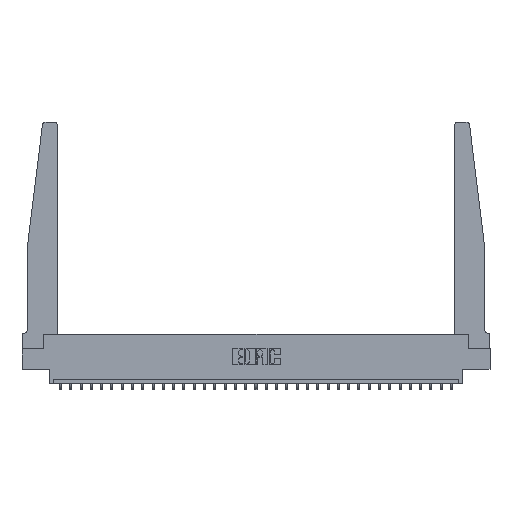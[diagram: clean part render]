
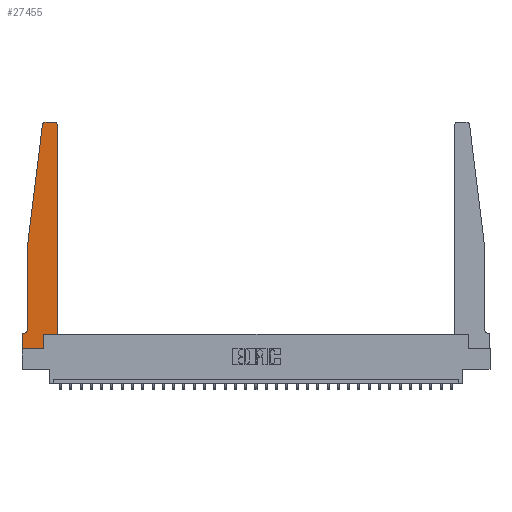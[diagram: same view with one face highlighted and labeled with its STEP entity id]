
A CAD part, top view. The second image highlights one B-rep face of the part: STEP entity #27455.
In plain terms, the highlighted planar face has unit normal (0, 0, 1).
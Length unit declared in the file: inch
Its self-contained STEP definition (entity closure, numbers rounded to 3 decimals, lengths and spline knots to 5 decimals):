
#43 = CARTESIAN_POINT ( 'NONE',  ( 0.065, 0.2375, 0.37 ) ) ;
#431 = CARTESIAN_POINT ( 'NONE',  ( 0.2605, 0., 0.37 ) ) ;
#449 = CARTESIAN_POINT ( 'NONE',  ( 0.395, 2.72, 0.37 ) ) ;
#1657 = AXIS2_PLACEMENT_3D ( 'NONE', #6123, #22128, #8421 ) ;
#2112 = CARTESIAN_POINT ( 'NONE',  ( 0.395, 2.75, 0.37 ) ) ;
#2204 = PLANE ( 'NONE',  #16980 ) ;
#2586 = CARTESIAN_POINT ( 'NONE',  ( 0.015, 0.2375, 0.37 ) ) ;
#2654 = DIRECTION ( 'NONE',  ( 0., -1., 0. ) ) ;
#2761 = DIRECTION ( 'NONE',  ( 1., 0., 0. ) ) ;
#3505 = VERTEX_POINT ( 'NONE', #2112 ) ;
#3593 = DIRECTION ( 'NONE',  ( 1., 0., 0. ) ) ;
#3623 = ORIENTED_EDGE ( 'NONE', *, *, #20259, .T. ) ;
#3693 = CARTESIAN_POINT ( 'NONE',  ( 0.425, 0.18, 0.37 ) ) ;
#3745 = CARTESIAN_POINT ( 'NONE',  ( 0.425, 2.72, 0.37 ) ) ;
#3950 = LINE ( 'NONE', #18635, #22200 ) ;
#3985 = EDGE_LOOP ( 'NONE', ( #28343, #24092, #12343, #15617, #10649, #20287, #22351, #16852, #3623, #20044, #4111, #4982 ) ) ;
#4071 = VERTEX_POINT ( 'NONE', #15637 ) ;
#4111 = ORIENTED_EDGE ( 'NONE', *, *, #15782, .T. ) ;
#4496 = EDGE_CURVE ( 'NONE', #15109, #15388, #22783, .T. ) ;
#4830 = DIRECTION ( 'NONE',  ( -1., 0., 0. ) ) ;
#4880 = VECTOR ( 'NONE', #12993, 39.37008 ) ;
#4982 = ORIENTED_EDGE ( 'NONE', *, *, #11538, .T. ) ;
#5104 = EDGE_CURVE ( 'NONE', #25351, #8278, #6281, .T. ) ;
#5552 = VERTEX_POINT ( 'NONE', #13343 ) ;
#5752 = CARTESIAN_POINT ( 'NONE',  ( 0., 0., 0.37 ) ) ;
#6123 = CARTESIAN_POINT ( 'NONE',  ( 0.27653, 2.72, 0.37 ) ) ;
#6281 = CIRCLE ( 'NONE', #25592, 0.05 ) ;
#6567 = LINE ( 'NONE', #28541, #11937 ) ;
#6596 = LINE ( 'NONE', #3693, #16604 ) ;
#6695 = VERTEX_POINT ( 'NONE', #15187 ) ;
#6770 = DIRECTION ( 'NONE',  ( 0., 0., 1. ) ) ;
#6935 = DIRECTION ( 'NONE',  ( -0.122, -0.992, 0. ) ) ;
#6980 = CARTESIAN_POINT ( 'NONE',  ( 0.2605, 0.18, 0.37 ) ) ;
#7722 = CARTESIAN_POINT ( 'NONE',  ( 0., 0.1875, 0.37 ) ) ;
#7790 = EDGE_CURVE ( 'NONE', #15388, #5552, #26459, .T. ) ;
#8278 = VERTEX_POINT ( 'NONE', #27007 ) ;
#8357 = DIRECTION ( 'NONE',  ( -1., 0., 0. ) ) ;
#8410 = CARTESIAN_POINT ( 'NONE',  ( 0.27653, 2.75, 0.37 ) ) ;
#8421 = DIRECTION ( 'NONE',  ( 1., 0., 0. ) ) ;
#8904 = EDGE_CURVE ( 'NONE', #11662, #17621, #9171, .T. ) ;
#9171 = LINE ( 'NONE', #29138, #21384 ) ;
#10018 = AXIS2_PLACEMENT_3D ( 'NONE', #449, #16435, #2761 ) ;
#10250 = DIRECTION ( 'NONE',  ( -1., 0., 0. ) ) ;
#10649 = ORIENTED_EDGE ( 'NONE', *, *, #5104, .T. ) ;
#11099 = EDGE_CURVE ( 'NONE', #8278, #11662, #6567, .T. ) ;
#11213 = EDGE_CURVE ( 'NONE', #3505, #15109, #21251, .T. ) ;
#11538 = EDGE_CURVE ( 'NONE', #25711, #3505, #13349, .T. ) ;
#11596 = DIRECTION ( 'NONE',  ( 0., 1., 0. ) ) ;
#11662 = VERTEX_POINT ( 'NONE', #7722 ) ;
#11937 = VECTOR ( 'NONE', #10250, 39.37008 ) ;
#12343 = ORIENTED_EDGE ( 'NONE', *, *, #7790, .T. ) ;
#12993 = DIRECTION ( 'NONE',  ( 0., 1., 0. ) ) ;
#13343 = CARTESIAN_POINT ( 'NONE',  ( 0.065, 1.25, 0.37 ) ) ;
#13349 = CIRCLE ( 'NONE', #10018, 0.03 ) ;
#13579 = VECTOR ( 'NONE', #6935, 39.37008 ) ;
#15109 = VERTEX_POINT ( 'NONE', #8410 ) ;
#15187 = CARTESIAN_POINT ( 'NONE',  ( 0.2605, 0.18, 0.37 ) ) ;
#15189 = CARTESIAN_POINT ( 'NONE',  ( 0.425, 0.18, 0.37 ) ) ;
#15388 = VERTEX_POINT ( 'NONE', #16288 ) ;
#15478 = DIRECTION ( 'NONE',  ( 0., -1., 0. ) ) ;
#15617 = ORIENTED_EDGE ( 'NONE', *, *, #28220, .T. ) ;
#15637 = CARTESIAN_POINT ( 'NONE',  ( 0.425, 0.18, 0.37 ) ) ;
#15782 = EDGE_CURVE ( 'NONE', #4071, #25711, #23158, .T. ) ;
#16288 = CARTESIAN_POINT ( 'NONE',  ( 0.24675, 2.72367, 0.37 ) ) ;
#16435 = DIRECTION ( 'NONE',  ( 0., 0., 1. ) ) ;
#16604 = VECTOR ( 'NONE', #3593, 39.37008 ) ;
#16852 = ORIENTED_EDGE ( 'NONE', *, *, #25065, .T. ) ;
#16980 = AXIS2_PLACEMENT_3D ( 'NONE', #20506, #6770, #22770 ) ;
#17393 = EDGE_CURVE ( 'NONE', #6695, #4071, #6596, .T. ) ;
#17621 = VERTEX_POINT ( 'NONE', #25154 ) ;
#17968 = FACE_OUTER_BOUND ( 'NONE', #3985, .T. ) ;
#18361 = CARTESIAN_POINT ( 'NONE',  ( 0.065, 1.25, 0.37 ) ) ;
#18571 = DIRECTION ( 'NONE',  ( 0., 0., -1. ) ) ;
#18635 = CARTESIAN_POINT ( 'NONE',  ( 0.065, 1.25, 0.37 ) ) ;
#19577 = DIRECTION ( 'NONE',  ( 1., 0., 0. ) ) ;
#20044 = ORIENTED_EDGE ( 'NONE', *, *, #17393, .T. ) ;
#20259 = EDGE_CURVE ( 'NONE', #28251, #6695, #28446, .T. ) ;
#20287 = ORIENTED_EDGE ( 'NONE', *, *, #11099, .T. ) ;
#20506 = CARTESIAN_POINT ( 'NONE',  ( 0., 0.1875, 0.37 ) ) ;
#21251 = LINE ( 'NONE', #24381, #27303 ) ;
#21384 = VECTOR ( 'NONE', #15478, 39.37008 ) ;
#22128 = DIRECTION ( 'NONE',  ( 0., 0., 1. ) ) ;
#22200 = VECTOR ( 'NONE', #2654, 39.37008 ) ;
#22351 = ORIENTED_EDGE ( 'NONE', *, *, #8904, .T. ) ;
#22398 = VECTOR ( 'NONE', #11596, 39.37008 ) ;
#22750 = LINE ( 'NONE', #5752, #28192 ) ;
#22770 = DIRECTION ( 'NONE',  ( 1., 0., 0. ) ) ;
#22783 = CIRCLE ( 'NONE', #1657, 0.03 ) ;
#23158 = LINE ( 'NONE', #15189, #4880 ) ;
#24092 = ORIENTED_EDGE ( 'NONE', *, *, #4496, .T. ) ;
#24381 = CARTESIAN_POINT ( 'NONE',  ( 0.25, 2.75, 0.37 ) ) ;
#25065 = EDGE_CURVE ( 'NONE', #17621, #28251, #22750, .T. ) ;
#25154 = CARTESIAN_POINT ( 'NONE',  ( 0., 0., 0.37 ) ) ;
#25351 = VERTEX_POINT ( 'NONE', #43 ) ;
#25592 = AXIS2_PLACEMENT_3D ( 'NONE', #2586, #18571, #4830 ) ;
#25711 = VERTEX_POINT ( 'NONE', #3745 ) ;
#26459 = LINE ( 'NONE', #18361, #13579 ) ;
#27007 = CARTESIAN_POINT ( 'NONE',  ( 0.015, 0.1875, 0.37 ) ) ;
#27303 = VECTOR ( 'NONE', #8357, 39.37008 ) ;
#27455 = ADVANCED_FACE ( 'NONE', ( #17968 ), #2204, .T. ) ;
#28192 = VECTOR ( 'NONE', #19577, 39.37008 ) ;
#28220 = EDGE_CURVE ( 'NONE', #5552, #25351, #3950, .T. ) ;
#28251 = VERTEX_POINT ( 'NONE', #431 ) ;
#28343 = ORIENTED_EDGE ( 'NONE', *, *, #11213, .T. ) ;
#28446 = LINE ( 'NONE', #6980, #22398 ) ;
#28541 = CARTESIAN_POINT ( 'NONE',  ( 0.065, 0.1875, 0.37 ) ) ;
#29138 = CARTESIAN_POINT ( 'NONE',  ( 0., 0., 0.37 ) ) ;
